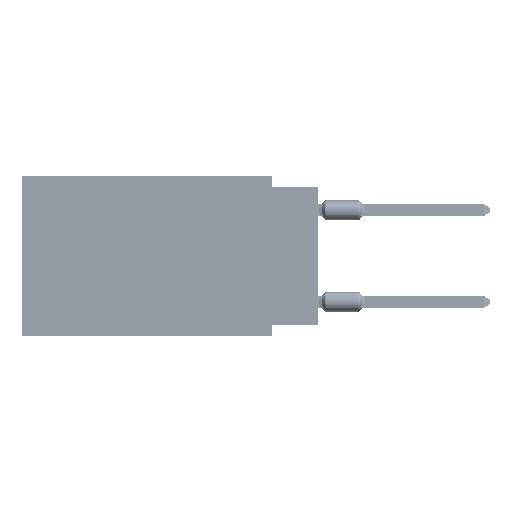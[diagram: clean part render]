
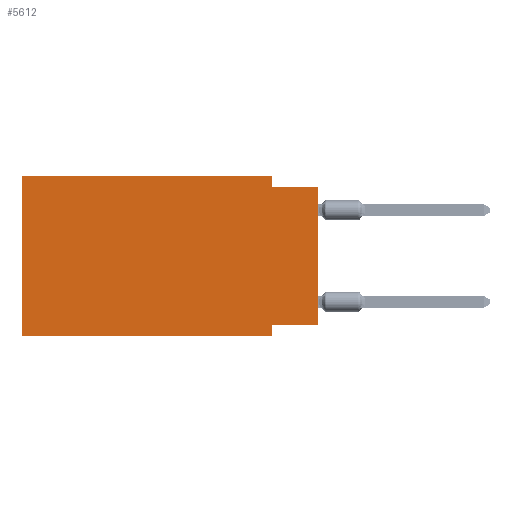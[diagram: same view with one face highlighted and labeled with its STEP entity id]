
A CAD part, left-side view. The second image highlights one B-rep face of the part: STEP entity #5612.
In plain terms, the highlighted planar face has unit normal (-1, 0, 0).
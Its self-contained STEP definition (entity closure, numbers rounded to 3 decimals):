
#43 = EDGE_CURVE ( 'NONE', #13925, #202, #75751, .T. ) ;
#202 = VERTEX_POINT ( 'NONE', #77745 ) ;
#1816 = LINE ( 'NONE', #52446, #72756 ) ;
#3941 = LINE ( 'NONE', #53351, #70774 ) ;
#4247 = ORIENTED_EDGE ( 'NONE', *, *, #20485, .F. ) ;
#5612 = ADVANCED_FACE ( 'NONE', ( #21914 ), #20715, .F. ) ;
#9032 = CARTESIAN_POINT ( 'NONE',  ( 0., 0., -0.635 ) ) ;
#10075 = VERTEX_POINT ( 'NONE', #70656 ) ;
#10416 = ORIENTED_EDGE ( 'NONE', *, *, #41962, .F. ) ;
#12050 = LINE ( 'NONE', #35952, #24677 ) ;
#12506 = CARTESIAN_POINT ( 'NONE',  ( 0., 2.54, -8.255 ) ) ;
#13452 = CARTESIAN_POINT ( 'NONE',  ( 0., 16.383, 0. ) ) ;
#13925 = VERTEX_POINT ( 'NONE', #32827 ) ;
#14839 = ORIENTED_EDGE ( 'NONE', *, *, #39792, .F. ) ;
#15774 = AXIS2_PLACEMENT_3D ( 'NONE', #70061, #22313, #39732 ) ;
#18535 = VECTOR ( 'NONE', #46448, 1000. ) ;
#18633 = ORIENTED_EDGE ( 'NONE', *, *, #43, .F. ) ;
#20485 = EDGE_CURVE ( 'NONE', #202, #24473, #27931, .T. ) ;
#20715 = PLANE ( 'NONE',  #15774 ) ;
#21783 = EDGE_CURVE ( 'NONE', #24473, #56357, #28443, .T. ) ;
#21914 = FACE_OUTER_BOUND ( 'NONE', #48186, .T. ) ;
#22313 = DIRECTION ( 'NONE',  ( 1., 0., 0. ) ) ;
#24473 = VERTEX_POINT ( 'NONE', #39282 ) ;
#24677 = VECTOR ( 'NONE', #36757, 1000. ) ;
#25095 = ORIENTED_EDGE ( 'NONE', *, *, #52365, .F. ) ;
#27245 = DIRECTION ( 'NONE',  ( 0., -1., 0. ) ) ;
#27398 = CARTESIAN_POINT ( 'NONE',  ( 0., 0., 0. ) ) ;
#27931 = LINE ( 'NONE', #65937, #29390 ) ;
#28443 = LINE ( 'NONE', #9032, #30904 ) ;
#28905 = DIRECTION ( 'NONE',  ( 0., 0., -1. ) ) ;
#29390 = VECTOR ( 'NONE', #35996, 1000. ) ;
#30904 = VECTOR ( 'NONE', #27245, 1000. ) ;
#31507 = CARTESIAN_POINT ( 'NONE',  ( 0., 16.383, -8.89 ) ) ;
#32812 = EDGE_CURVE ( 'NONE', #10075, #56357, #77538, .T. ) ;
#32827 = CARTESIAN_POINT ( 'NONE',  ( 0., 16.383, 0. ) ) ;
#34333 = EDGE_CURVE ( 'NONE', #77526, #69669, #1816, .T. ) ;
#35952 = CARTESIAN_POINT ( 'NONE',  ( 0., 16.383, 0. ) ) ;
#35996 = DIRECTION ( 'NONE',  ( 0., 0., -1. ) ) ;
#36001 = VECTOR ( 'NONE', #38563, 1000. ) ;
#36757 = DIRECTION ( 'NONE',  ( 0., 0., 1. ) ) ;
#38563 = DIRECTION ( 'NONE',  ( 0., -1., 0. ) ) ;
#39282 = CARTESIAN_POINT ( 'NONE',  ( 0., 2.54, -0.635 ) ) ;
#39732 = DIRECTION ( 'NONE',  ( 0., 0., -1. ) ) ;
#39792 = EDGE_CURVE ( 'NONE', #77526, #13925, #12050, .T. ) ;
#41196 = DIRECTION ( 'NONE',  ( 0., 1., 0. ) ) ;
#41458 = CARTESIAN_POINT ( 'NONE',  ( 0., 2.54, -8.89 ) ) ;
#41502 = CARTESIAN_POINT ( 'NONE',  ( 0., 0., -0.635 ) ) ;
#41962 = EDGE_CURVE ( 'NONE', #62784, #69669, #78245, .T. ) ;
#46448 = DIRECTION ( 'NONE',  ( 0., 0., 1. ) ) ;
#47304 = ORIENTED_EDGE ( 'NONE', *, *, #32812, .T. ) ;
#47514 = ORIENTED_EDGE ( 'NONE', *, *, #21783, .F. ) ;
#48186 = EDGE_LOOP ( 'NONE', ( #47304, #47514, #4247, #18633, #14839, #54064, #10416, #25095 ) ) ;
#51241 = DIRECTION ( 'NONE',  ( 0., -1., 0. ) ) ;
#52365 = EDGE_CURVE ( 'NONE', #10075, #62784, #3941, .T. ) ;
#52446 = CARTESIAN_POINT ( 'NONE',  ( 0., 16.383, -8.89 ) ) ;
#53351 = CARTESIAN_POINT ( 'NONE',  ( 0., 0., -8.255 ) ) ;
#54064 = ORIENTED_EDGE ( 'NONE', *, *, #34333, .T. ) ;
#56357 = VERTEX_POINT ( 'NONE', #41502 ) ;
#62784 = VERTEX_POINT ( 'NONE', #12506 ) ;
#65937 = CARTESIAN_POINT ( 'NONE',  ( 0., 2.54, 0. ) ) ;
#67579 = VECTOR ( 'NONE', #28905, 1000. ) ;
#69669 = VERTEX_POINT ( 'NONE', #70865 ) ;
#70061 = CARTESIAN_POINT ( 'NONE',  ( 0., 16.383, 0. ) ) ;
#70656 = CARTESIAN_POINT ( 'NONE',  ( 0., 0., -8.255 ) ) ;
#70774 = VECTOR ( 'NONE', #41196, 1000. ) ;
#70865 = CARTESIAN_POINT ( 'NONE',  ( 0., 2.54, -8.89 ) ) ;
#72756 = VECTOR ( 'NONE', #51241, 1000. ) ;
#75751 = LINE ( 'NONE', #13452, #36001 ) ;
#77526 = VERTEX_POINT ( 'NONE', #31507 ) ;
#77538 = LINE ( 'NONE', #27398, #18535 ) ;
#77745 = CARTESIAN_POINT ( 'NONE',  ( 0., 2.54, 0. ) ) ;
#78245 = LINE ( 'NONE', #41458, #67579 ) ;
